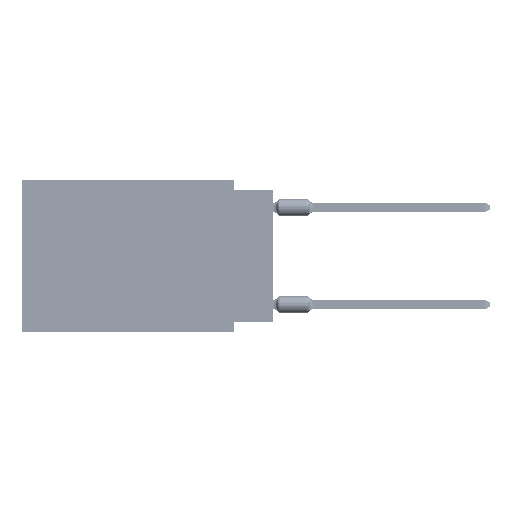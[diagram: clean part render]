
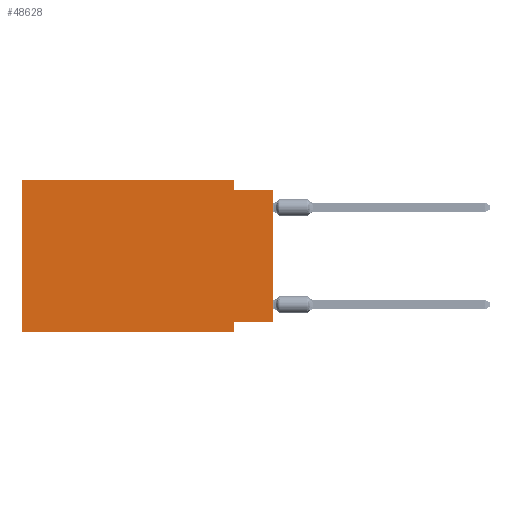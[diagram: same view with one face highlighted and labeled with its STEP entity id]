
A CAD part, left-side view. The second image highlights one B-rep face of the part: STEP entity #48628.
In plain terms, the highlighted planar face has unit normal (-1, 0, 0).
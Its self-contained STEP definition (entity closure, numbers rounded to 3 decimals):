
#1397 = DIRECTION ( 'NONE',  ( 0., 0., -1. ) ) ;
#1910 = ORIENTED_EDGE ( 'NONE', *, *, #34420, .F. ) ;
#2302 = LINE ( 'NONE', #15780, #19423 ) ;
#3034 = ORIENTED_EDGE ( 'NONE', *, *, #62104, .T. ) ;
#3558 = CARTESIAN_POINT ( 'NONE',  ( 0., 16.383, 0. ) ) ;
#4008 = FACE_OUTER_BOUND ( 'NONE', #24144, .T. ) ;
#4120 = LINE ( 'NONE', #31472, #37153 ) ;
#5319 = CARTESIAN_POINT ( 'NONE',  ( 0., 0., 0. ) ) ;
#5443 = DIRECTION ( 'NONE',  ( 0., 0., -1. ) ) ;
#6272 = VERTEX_POINT ( 'NONE', #54541 ) ;
#7662 = LINE ( 'NONE', #68189, #20912 ) ;
#9260 = CARTESIAN_POINT ( 'NONE',  ( 0., 16.383, 0. ) ) ;
#12912 = EDGE_CURVE ( 'NONE', #6272, #16971, #39964, .T. ) ;
#15780 = CARTESIAN_POINT ( 'NONE',  ( 0., 16.383, 0. ) ) ;
#16971 = VERTEX_POINT ( 'NONE', #57562 ) ;
#17897 = PLANE ( 'NONE',  #21800 ) ;
#19423 = VECTOR ( 'NONE', #23801, 1000. ) ;
#20443 = CARTESIAN_POINT ( 'NONE',  ( 0., 16.383, -9.906 ) ) ;
#20912 = VECTOR ( 'NONE', #1397, 1000. ) ;
#21800 = AXIS2_PLACEMENT_3D ( 'NONE', #3558, #23742, #66740 ) ;
#23742 = DIRECTION ( 'NONE',  ( 1., 0., 0. ) ) ;
#23801 = DIRECTION ( 'NONE',  ( 0., 0., 1. ) ) ;
#24144 = EDGE_LOOP ( 'NONE', ( #86258, #54867, #32589, #86892, #1910, #3034, #73667, #28192 ) ) ;
#25943 = DIRECTION ( 'NONE',  ( 0., 0., 1. ) ) ;
#28192 = ORIENTED_EDGE ( 'NONE', *, *, #12912, .F. ) ;
#29130 = CARTESIAN_POINT ( 'NONE',  ( 0., 2.54, -9.906 ) ) ;
#30510 = CARTESIAN_POINT ( 'NONE',  ( 0., 16.383, -9.906 ) ) ;
#31472 = CARTESIAN_POINT ( 'NONE',  ( 0., 2.54, -9.906 ) ) ;
#32589 = ORIENTED_EDGE ( 'NONE', *, *, #64159, .F. ) ;
#33719 = VECTOR ( 'NONE', #25943, 1000. ) ;
#34420 = EDGE_CURVE ( 'NONE', #40103, #36451, #2302, .T. ) ;
#36451 = VERTEX_POINT ( 'NONE', #9260 ) ;
#37153 = VECTOR ( 'NONE', #5443, 1000. ) ;
#38760 = CARTESIAN_POINT ( 'NONE',  ( 0., 2.54, 0. ) ) ;
#39964 = LINE ( 'NONE', #81196, #85551 ) ;
#40103 = VERTEX_POINT ( 'NONE', #30510 ) ;
#40740 = DIRECTION ( 'NONE',  ( 0., -1., 0. ) ) ;
#41493 = VECTOR ( 'NONE', #40740, 1000. ) ;
#42836 = CARTESIAN_POINT ( 'NONE',  ( 0., 0., -0.635 ) ) ;
#45122 = VERTEX_POINT ( 'NONE', #42836 ) ;
#48628 = ADVANCED_FACE ( 'NONE', ( #4008 ), #17897, .F. ) ;
#49447 = CARTESIAN_POINT ( 'NONE',  ( 0., 2.54, -0.635 ) ) ;
#51522 = LINE ( 'NONE', #72137, #62515 ) ;
#54541 = CARTESIAN_POINT ( 'NONE',  ( 0., 0., -9.271 ) ) ;
#54867 = ORIENTED_EDGE ( 'NONE', *, *, #85691, .F. ) ;
#57562 = CARTESIAN_POINT ( 'NONE',  ( 0., 2.54, -9.271 ) ) ;
#57721 = EDGE_CURVE ( 'NONE', #16971, #73377, #4120, .T. ) ;
#59439 = EDGE_CURVE ( 'NONE', #36451, #71838, #83326, .T. ) ;
#60476 = VERTEX_POINT ( 'NONE', #49447 ) ;
#62104 = EDGE_CURVE ( 'NONE', #40103, #73377, #75571, .T. ) ;
#62515 = VECTOR ( 'NONE', #65862, 1000. ) ;
#64159 = EDGE_CURVE ( 'NONE', #71838, #60476, #7662, .T. ) ;
#65862 = DIRECTION ( 'NONE',  ( 0., -1., 0. ) ) ;
#66280 = LINE ( 'NONE', #5319, #33719 ) ;
#66740 = DIRECTION ( 'NONE',  ( 0., 0., -1. ) ) ;
#68189 = CARTESIAN_POINT ( 'NONE',  ( 0., 2.54, 0. ) ) ;
#69261 = DIRECTION ( 'NONE',  ( 0., -1., 0. ) ) ;
#71838 = VERTEX_POINT ( 'NONE', #38760 ) ;
#72137 = CARTESIAN_POINT ( 'NONE',  ( 0., 0., -0.635 ) ) ;
#73132 = DIRECTION ( 'NONE',  ( 0., 1., 0. ) ) ;
#73377 = VERTEX_POINT ( 'NONE', #29130 ) ;
#73667 = ORIENTED_EDGE ( 'NONE', *, *, #57721, .F. ) ;
#75571 = LINE ( 'NONE', #20443, #80449 ) ;
#80449 = VECTOR ( 'NONE', #69261, 1000. ) ;
#81196 = CARTESIAN_POINT ( 'NONE',  ( 0., 0., -9.271 ) ) ;
#82000 = CARTESIAN_POINT ( 'NONE',  ( 0., 16.383, 0. ) ) ;
#83326 = LINE ( 'NONE', #82000, #41493 ) ;
#84082 = EDGE_CURVE ( 'NONE', #6272, #45122, #66280, .T. ) ;
#85551 = VECTOR ( 'NONE', #73132, 1000. ) ;
#85691 = EDGE_CURVE ( 'NONE', #60476, #45122, #51522, .T. ) ;
#86258 = ORIENTED_EDGE ( 'NONE', *, *, #84082, .T. ) ;
#86892 = ORIENTED_EDGE ( 'NONE', *, *, #59439, .F. ) ;
